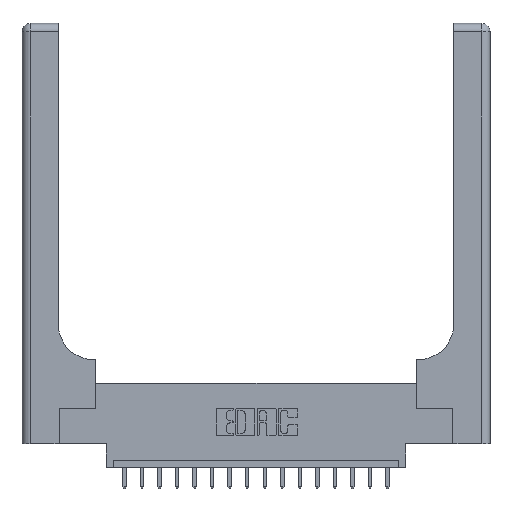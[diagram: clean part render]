
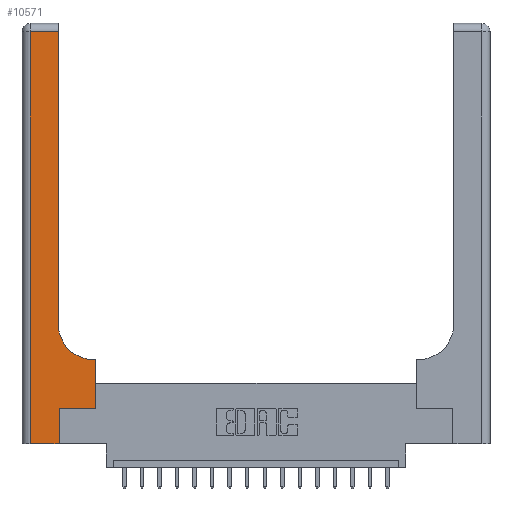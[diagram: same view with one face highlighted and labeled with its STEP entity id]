
A CAD part, top view. The second image highlights one B-rep face of the part: STEP entity #10571.
In plain terms, the highlighted planar face has unit normal (0, 0, 1).
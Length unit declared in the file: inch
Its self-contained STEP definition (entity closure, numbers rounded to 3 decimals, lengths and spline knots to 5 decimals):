
#51 = LINE ( 'NONE', #7861, #1130 ) ;
#312 = EDGE_CURVE ( 'NONE', #11644, #4208, #10004, .T. ) ;
#496 = DIRECTION ( 'NONE',  ( -1., 0., 0. ) ) ;
#871 = AXIS2_PLACEMENT_3D ( 'NONE', #12394, #15406, #496 ) ;
#1058 = DIRECTION ( 'NONE',  ( 0., 1., 0. ) ) ;
#1130 = VECTOR ( 'NONE', #13774, 39.37008 ) ;
#1241 = ORIENTED_EDGE ( 'NONE', *, *, #6937, .T. ) ;
#1250 = VERTEX_POINT ( 'NONE', #18601 ) ;
#1349 = ORIENTED_EDGE ( 'NONE', *, *, #17129, .T. ) ;
#1404 = CARTESIAN_POINT ( 'NONE',  ( 0.265, 0., 0.37 ) ) ;
#1641 = ORIENTED_EDGE ( 'NONE', *, *, #13235, .T. ) ;
#2360 = EDGE_CURVE ( 'NONE', #8423, #4023, #10036, .T. ) ;
#2653 = CARTESIAN_POINT ( 'NONE',  ( 0.265, 0., 0.37 ) ) ;
#2706 = DIRECTION ( 'NONE',  ( -1., 0., 0. ) ) ;
#2930 = ORIENTED_EDGE ( 'NONE', *, *, #18246, .T. ) ;
#3452 = VECTOR ( 'NONE', #12896, 39.37008 ) ;
#3462 = CARTESIAN_POINT ( 'NONE',  ( 0.528, 0.25, 0.37 ) ) ;
#3496 = ORIENTED_EDGE ( 'NONE', *, *, #2360, .T. ) ;
#3598 = VERTEX_POINT ( 'NONE', #3462 ) ;
#3901 = CARTESIAN_POINT ( 'NONE',  ( 0., 0., 0.37 ) ) ;
#3957 = ORIENTED_EDGE ( 'NONE', *, *, #16739, .T. ) ;
#4023 = VERTEX_POINT ( 'NONE', #7971 ) ;
#4188 = LINE ( 'NONE', #3901, #3452 ) ;
#4208 = VERTEX_POINT ( 'NONE', #10089 ) ;
#4225 = LINE ( 'NONE', #7212, #11156 ) ;
#4821 = CARTESIAN_POINT ( 'NONE',  ( 0.26, 2.94, 0.37 ) ) ;
#4835 = VERTEX_POINT ( 'NONE', #4821 ) ;
#5031 = EDGE_CURVE ( 'NONE', #4835, #11644, #4225, .T. ) ;
#5260 = CARTESIAN_POINT ( 'NONE',  ( 0.51, 0.85, 0.37 ) ) ;
#5401 = ORIENTED_EDGE ( 'NONE', *, *, #12959, .T. ) ;
#5799 = VECTOR ( 'NONE', #8367, 39.37008 ) ;
#6347 = AXIS2_PLACEMENT_3D ( 'NONE', #5260, #14148, #17192 ) ;
#6937 = EDGE_CURVE ( 'NONE', #4208, #15344, #4188, .T. ) ;
#7212 = CARTESIAN_POINT ( 'NONE',  ( 0., 2.94, 0.37 ) ) ;
#7247 = VECTOR ( 'NONE', #2706, 39.37008 ) ;
#7782 = ORIENTED_EDGE ( 'NONE', *, *, #5031, .T. ) ;
#7861 = CARTESIAN_POINT ( 'NONE',  ( 0.26, 3., 0.37 ) ) ;
#7971 = CARTESIAN_POINT ( 'NONE',  ( 0.51, 0.6, 0.37 ) ) ;
#8029 = PLANE ( 'NONE',  #871 ) ;
#8295 = CARTESIAN_POINT ( 'NONE',  ( 0.528, 0.25, 0.37 ) ) ;
#8367 = DIRECTION ( 'NONE',  ( 0., -1., 0. ) ) ;
#8423 = VERTEX_POINT ( 'NONE', #14927 ) ;
#8571 = DIRECTION ( 'NONE',  ( -1., 0., 0. ) ) ;
#9243 = ORIENTED_EDGE ( 'NONE', *, *, #312, .T. ) ;
#9273 = VECTOR ( 'NONE', #14910, 39.37008 ) ;
#9423 = VECTOR ( 'NONE', #18974, 39.37008 ) ;
#10004 = LINE ( 'NONE', #10102, #5799 ) ;
#10036 = LINE ( 'NONE', #14701, #7247 ) ;
#10089 = CARTESIAN_POINT ( 'NONE',  ( 0.06, 0., 0.37 ) ) ;
#10093 = LINE ( 'NONE', #1404, #9423 ) ;
#10102 = CARTESIAN_POINT ( 'NONE',  ( 0.06, 3., 0.37 ) ) ;
#10320 = CARTESIAN_POINT ( 'NONE',  ( 0.265, 0.25, 0.37 ) ) ;
#10571 = ADVANCED_FACE ( 'NONE', ( #16415 ), #8029, .F. ) ;
#11156 = VECTOR ( 'NONE', #8571, 39.37008 ) ;
#11644 = VERTEX_POINT ( 'NONE', #12643 ) ;
#12394 = CARTESIAN_POINT ( 'NONE',  ( 0., 3., 0.37 ) ) ;
#12643 = CARTESIAN_POINT ( 'NONE',  ( 0.06, 2.94, 0.37 ) ) ;
#12896 = DIRECTION ( 'NONE',  ( 1., 0., 0. ) ) ;
#12959 = EDGE_CURVE ( 'NONE', #18200, #3598, #16586, .T. ) ;
#13235 = EDGE_CURVE ( 'NONE', #3598, #8423, #18811, .T. ) ;
#13314 = VECTOR ( 'NONE', #1058, 39.37008 ) ;
#13774 = DIRECTION ( 'NONE',  ( 0., 1., 0. ) ) ;
#14148 = DIRECTION ( 'NONE',  ( 0., 0., -1. ) ) ;
#14701 = CARTESIAN_POINT ( 'NONE',  ( 0.26, 0.6, 0.37 ) ) ;
#14910 = DIRECTION ( 'NONE',  ( 1., 0., 0. ) ) ;
#14927 = CARTESIAN_POINT ( 'NONE',  ( 0.528, 0.6, 0.37 ) ) ;
#15344 = VERTEX_POINT ( 'NONE', #2653 ) ;
#15406 = DIRECTION ( 'NONE',  ( 0., 0., -1. ) ) ;
#16415 = FACE_OUTER_BOUND ( 'NONE', #18231, .T. ) ;
#16494 = CARTESIAN_POINT ( 'NONE',  ( 0.265, 0.25, 0.37 ) ) ;
#16586 = LINE ( 'NONE', #16494, #9273 ) ;
#16593 = CIRCLE ( 'NONE', #6347, 0.25 ) ;
#16739 = EDGE_CURVE ( 'NONE', #15344, #18200, #10093, .T. ) ;
#17129 = EDGE_CURVE ( 'NONE', #4023, #1250, #16593, .T. ) ;
#17192 = DIRECTION ( 'NONE',  ( 1., 0., 0. ) ) ;
#18200 = VERTEX_POINT ( 'NONE', #10320 ) ;
#18231 = EDGE_LOOP ( 'NONE', ( #2930, #7782, #9243, #1241, #3957, #5401, #1641, #3496, #1349 ) ) ;
#18246 = EDGE_CURVE ( 'NONE', #1250, #4835, #51, .T. ) ;
#18601 = CARTESIAN_POINT ( 'NONE',  ( 0.26, 0.85, 0.37 ) ) ;
#18811 = LINE ( 'NONE', #8295, #13314 ) ;
#18974 = DIRECTION ( 'NONE',  ( 0., 1., 0. ) ) ;
